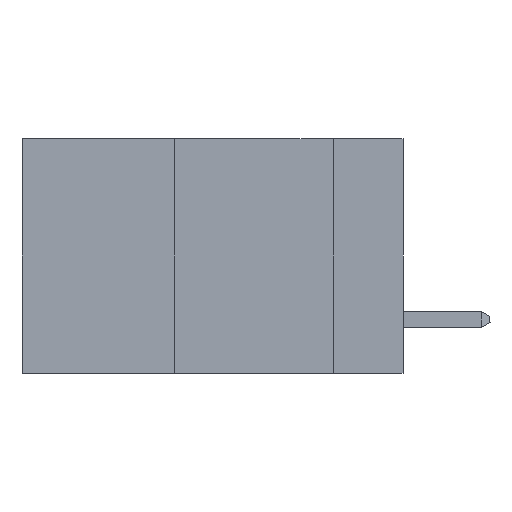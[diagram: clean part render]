
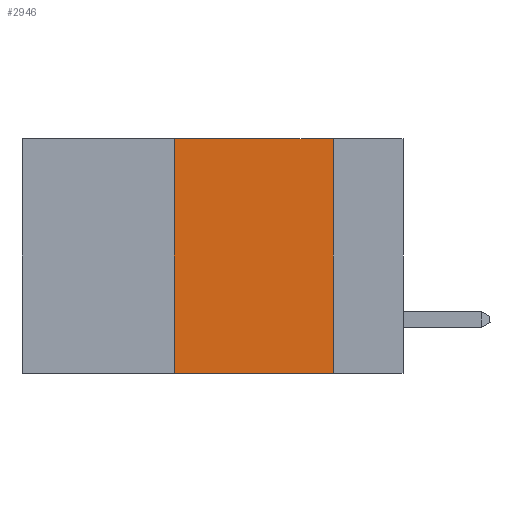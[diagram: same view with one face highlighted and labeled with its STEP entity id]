
A CAD part, left-side view. The second image highlights one B-rep face of the part: STEP entity #2946.
In plain terms, the highlighted planar face has unit normal (-1, 0, 0).
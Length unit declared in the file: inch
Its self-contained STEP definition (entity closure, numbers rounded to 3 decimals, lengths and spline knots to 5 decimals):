
#269 = EDGE_LOOP ( 'NONE', ( #511, #12455, #26441, #16064 ) ) ;
#511 = ORIENTED_EDGE ( 'NONE', *, *, #12627, .F. ) ;
#1494 = CARTESIAN_POINT ( 'NONE',  ( 0., 0.36, 0. ) ) ;
#1500 = EDGE_CURVE ( 'NONE', #28991, #35277, #21437, .T. ) ;
#2946 = ADVANCED_FACE ( 'NONE', ( #16527 ), #41566, .F. ) ;
#4033 = EDGE_CURVE ( 'NONE', #35814, #17275, #41498, .T. ) ;
#5229 = VECTOR ( 'NONE', #27870, 39.37008 ) ;
#5889 = CARTESIAN_POINT ( 'NONE',  ( 0., 0.36, 0. ) ) ;
#8499 = DIRECTION ( 'NONE',  ( 0., 0., 1. ) ) ;
#9408 = DIRECTION ( 'NONE',  ( 0., -1., 0. ) ) ;
#12455 = ORIENTED_EDGE ( 'NONE', *, *, #1500, .F. ) ;
#12627 = EDGE_CURVE ( 'NONE', #35277, #17275, #44056, .T. ) ;
#16064 = ORIENTED_EDGE ( 'NONE', *, *, #4033, .T. ) ;
#16527 = FACE_OUTER_BOUND ( 'NONE', #269, .T. ) ;
#17275 = VERTEX_POINT ( 'NONE', #23527 ) ;
#20620 = CARTESIAN_POINT ( 'NONE',  ( 0., 0.6, 0. ) ) ;
#21437 = LINE ( 'NONE', #35185, #5229 ) ;
#23191 = VECTOR ( 'NONE', #9408, 39.37008 ) ;
#23527 = CARTESIAN_POINT ( 'NONE',  ( 0., 0.11, -0.37 ) ) ;
#26441 = ORIENTED_EDGE ( 'NONE', *, *, #43549, .F. ) ;
#26530 = AXIS2_PLACEMENT_3D ( 'NONE', #20620, #31435, #31155 ) ;
#27870 = DIRECTION ( 'NONE',  ( 0., -1., 0. ) ) ;
#28304 = CARTESIAN_POINT ( 'NONE',  ( 0., 0.36, -0.37 ) ) ;
#28991 = VERTEX_POINT ( 'NONE', #5889 ) ;
#29925 = CARTESIAN_POINT ( 'NONE',  ( 0., 0.6, -0.37 ) ) ;
#31155 = DIRECTION ( 'NONE',  ( 0., 0., -1. ) ) ;
#31435 = DIRECTION ( 'NONE',  ( 1., 0., 0. ) ) ;
#32259 = CARTESIAN_POINT ( 'NONE',  ( 0., 0.11, 0. ) ) ;
#34806 = VECTOR ( 'NONE', #44697, 39.37008 ) ;
#35185 = CARTESIAN_POINT ( 'NONE',  ( 0., 0.6, 0. ) ) ;
#35277 = VERTEX_POINT ( 'NONE', #32259 ) ;
#35435 = VECTOR ( 'NONE', #8499, 39.37008 ) ;
#35814 = VERTEX_POINT ( 'NONE', #28304 ) ;
#40366 = LINE ( 'NONE', #1494, #35435 ) ;
#40498 = CARTESIAN_POINT ( 'NONE',  ( 0., 0.11, 0. ) ) ;
#41498 = LINE ( 'NONE', #29925, #23191 ) ;
#41566 = PLANE ( 'NONE',  #26530 ) ;
#43549 = EDGE_CURVE ( 'NONE', #35814, #28991, #40366, .T. ) ;
#44056 = LINE ( 'NONE', #40498, #34806 ) ;
#44697 = DIRECTION ( 'NONE',  ( 0., 0., -1. ) ) ;
